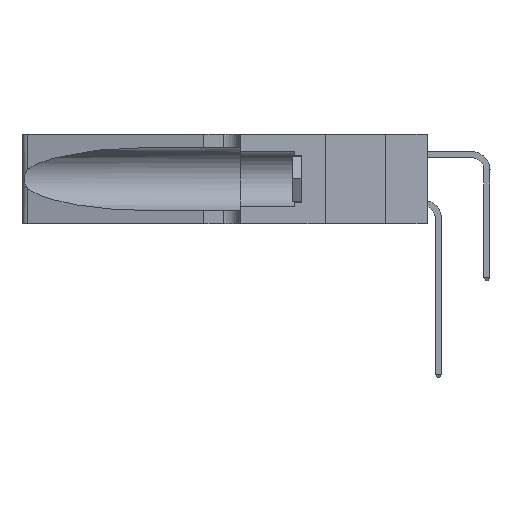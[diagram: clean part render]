
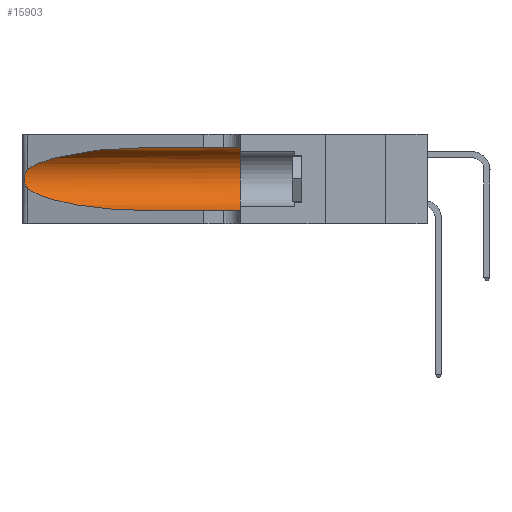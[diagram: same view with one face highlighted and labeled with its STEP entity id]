
A CAD part, left-side view. The second image highlights one B-rep face of the part: STEP entity #15903.
In plain terms, the highlighted cylindrical face has radius 3.308 mm (diameter 6.617 mm), a partial arc.
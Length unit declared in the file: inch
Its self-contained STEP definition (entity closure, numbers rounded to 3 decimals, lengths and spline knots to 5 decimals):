
#679 = EDGE_CURVE ( 'NONE', #4232, #12598, #23984, .T. ) ;
#851 = EDGE_CURVE ( 'NONE', #18237, #4232, #17004, .T. ) ;
#1203 = DIRECTION ( 'NONE',  ( 0., -1., 0. ) ) ;
#1647 = CARTESIAN_POINT ( 'NONE',  ( 0.26075, 1.23896, 0.178 ) ) ;
#2596 = CARTESIAN_POINT ( 'NONE',  ( 0.1305, 1.61858, 0.05475 ) ) ;
#2837 = CARTESIAN_POINT ( 'NONE',  ( 0.1305, 0.72297, 0.31525 ) ) ;
#2969 = CARTESIAN_POINT ( 'NONE',  ( 0.25487, 1.22718, 0.22369 ) ) ;
#3493 = DIRECTION ( 'NONE',  ( 0., 1., 0. ) ) ;
#4046 = CARTESIAN_POINT ( 'NONE',  ( 0.1305, 0.35, 0.31525 ) ) ;
#4232 = VERTEX_POINT ( 'NONE', #13724 ) ;
#4397 = ORIENTED_EDGE ( 'NONE', *, *, #5051, .T. ) ;
#4727 = CARTESIAN_POINT ( 'NONE',  ( 0.25856, 1.23593, 0.16098 ) ) ;
#5051 = EDGE_CURVE ( 'NONE', #12598, #11474, #25355, .T. ) ;
#6805 = CYLINDRICAL_SURFACE ( 'NONE', #19938, 0.13025 ) ;
#6908 = DIRECTION ( 'NONE',  ( 0., -1., 0. ) ) ;
#6914 = EDGE_CURVE ( 'NONE', #38770, #18237, #28026, .T. ) ;
#7745 = CARTESIAN_POINT ( 'NONE',  ( 0.25639, 1.23186, 0.15144 ) ) ;
#8310 = ORIENTED_EDGE ( 'NONE', *, *, #851, .T. ) ;
#8342 = VECTOR ( 'NONE', #6908, 39.37008 ) ;
#9471 = EDGE_CURVE ( 'NONE', #15850, #11474, #17674, .T. ) ;
#9672 = FACE_OUTER_BOUND ( 'NONE', #24500, .T. ) ;
#10287 = VECTOR ( 'NONE', #20826, 39.37008 ) ;
#10779 = CARTESIAN_POINT ( 'NONE',  ( 0.25487, 1.22718, 0.14631 ) ) ;
#11474 = VERTEX_POINT ( 'NONE', #18037 ) ;
#11837 = ORIENTED_EDGE ( 'NONE', *, *, #9471, .F. ) ;
#12598 = VERTEX_POINT ( 'NONE', #28041 ) ;
#12914 = CARTESIAN_POINT ( 'NONE',  ( 0.18966, 0.96281, 0.05475 ) ) ;
#13563 = CARTESIAN_POINT ( 'NONE',  ( 0.25487, 1.22718, 0.22369 ) ) ;
#13684 = CARTESIAN_POINT ( 'NONE',  ( 0.25639, 1.23184, 0.21858 ) ) ;
#13724 = CARTESIAN_POINT ( 'NONE',  ( 0.25487, 1.22718, 0.14631 ) ) ;
#15850 = VERTEX_POINT ( 'NONE', #4046 ) ;
#15903 = ADVANCED_FACE ( 'NONE', ( #9672 ), #6805, .F. ) ;
#15974 = CARTESIAN_POINT ( 'NONE',  ( 0.2373, 1.15595, 0.08982 ) ) ;
#16754 = CARTESIAN_POINT ( 'NONE',  ( 0.25854, 1.2359, 0.20912 ) ) ;
#17004 = B_SPLINE_CURVE_WITH_KNOTS ( 'NONE', 3,
 ( #13563, #25658, #13684, #34606, #16754, #37553, #19766, #1647, #22784, #4727, #25782, #7745, #28776, #10779 ),
 .UNSPECIFIED., .F., .F.,
 ( 4, 2, 2, 2, 2, 2, 4 ),
 ( 0., 0.00027, 0.00053, 0.00107, 0.0016, 0.00187, 0.00214 ),
 .UNSPECIFIED. ) ;
#17674 = CIRCLE ( 'NONE', #18701, 0.13025 ) ;
#18037 = CARTESIAN_POINT ( 'NONE',  ( 0.1305, 0.35, 0.05475 ) ) ;
#18051 = CARTESIAN_POINT ( 'NONE',  ( 0.18966, 0.96281, 0.31525 ) ) ;
#18237 = VERTEX_POINT ( 'NONE', #18646 ) ;
#18646 = CARTESIAN_POINT ( 'NONE',  ( 0.25487, 1.22718, 0.22369 ) ) ;
#18701 = AXIS2_PLACEMENT_3D ( 'NONE', #21568, #3493, #24568 ) ;
#19014 = CARTESIAN_POINT ( 'NONE',  ( 0.1305, 0.72297, 0.05475 ) ) ;
#19357 = CARTESIAN_POINT ( 'NONE',  ( 0.1305, 1.61858, 0.185 ) ) ;
#19766 = CARTESIAN_POINT ( 'NONE',  ( 0.26075, 1.23896, 0.19203 ) ) ;
#19938 = AXIS2_PLACEMENT_3D ( 'NONE', #19357, #1203, #25365 ) ;
#20826 = DIRECTION ( 'NONE',  ( 0., -1., 0. ) ) ;
#21058 = CARTESIAN_POINT ( 'NONE',  ( 0.2373, 1.15595, 0.28018 ) ) ;
#21088 = ORIENTED_EDGE ( 'NONE', *, *, #37718, .F. ) ;
#21568 = CARTESIAN_POINT ( 'NONE',  ( 0.1305, 0.35, 0.185 ) ) ;
#22784 = CARTESIAN_POINT ( 'NONE',  ( 0.26017, 1.23833, 0.17102 ) ) ;
#23112 = ORIENTED_EDGE ( 'NONE', *, *, #6914, .T. ) ;
#23612 = CARTESIAN_POINT ( 'NONE',  ( 0.1305, 0.72297, 0.31525 ) ) ;
#23984 =( BOUNDED_CURVE ( )  B_SPLINE_CURVE ( 3, ( #36796, #15974, #12914, #19014 ),
 .UNSPECIFIED., .F., .F. ) 
 B_SPLINE_CURVE_WITH_KNOTS ( ( 4, 4 ),
 ( 3.44316, 4.71239 ),
 .UNSPECIFIED. ) 
 CURVE ( )  GEOMETRIC_REPRESENTATION_ITEM ( )  RATIONAL_B_SPLINE_CURVE ( ( 1., 0.87, 0.87, 1. ) ) 
 REPRESENTATION_ITEM ( '' )  );
#24134 = ORIENTED_EDGE ( 'NONE', *, *, #679, .T. ) ;
#24386 = LINE ( 'NONE', #27961, #8342 ) ;
#24500 = EDGE_LOOP ( 'NONE', ( #23112, #8310, #24134, #4397, #11837, #21088 ) ) ;
#24568 = DIRECTION ( 'NONE',  ( 0., 0., 1. ) ) ;
#25355 = LINE ( 'NONE', #2596, #10287 ) ;
#25365 = DIRECTION ( 'NONE',  ( 0., 0., -1. ) ) ;
#25658 = CARTESIAN_POINT ( 'NONE',  ( 0.25555, 1.22994, 0.2215 ) ) ;
#25782 = CARTESIAN_POINT ( 'NONE',  ( 0.25789, 1.23486, 0.15765 ) ) ;
#27961 = CARTESIAN_POINT ( 'NONE',  ( 0.1305, 1.61858, 0.31525 ) ) ;
#28026 =( BOUNDED_CURVE ( )  B_SPLINE_CURVE ( 3, ( #2837, #18051, #21058, #2969 ),
 .UNSPECIFIED., .F., .F. ) 
 B_SPLINE_CURVE_WITH_KNOTS ( ( 4, 4 ),
 ( 1.5708, 2.84003 ),
 .UNSPECIFIED. ) 
 CURVE ( )  GEOMETRIC_REPRESENTATION_ITEM ( )  RATIONAL_B_SPLINE_CURVE ( ( 1., 0.87, 0.87, 1. ) ) 
 REPRESENTATION_ITEM ( '' )  );
#28041 = CARTESIAN_POINT ( 'NONE',  ( 0.1305, 0.72297, 0.05475 ) ) ;
#28776 = CARTESIAN_POINT ( 'NONE',  ( 0.25555, 1.22993, 0.14849 ) ) ;
#34606 = CARTESIAN_POINT ( 'NONE',  ( 0.25787, 1.23484, 0.2124 ) ) ;
#36796 = CARTESIAN_POINT ( 'NONE',  ( 0.25487, 1.22718, 0.14631 ) ) ;
#37553 = CARTESIAN_POINT ( 'NONE',  ( 0.26018, 1.23835, 0.19895 ) ) ;
#37718 = EDGE_CURVE ( 'NONE', #38770, #15850, #24386, .T. ) ;
#38770 = VERTEX_POINT ( 'NONE', #23612 ) ;
